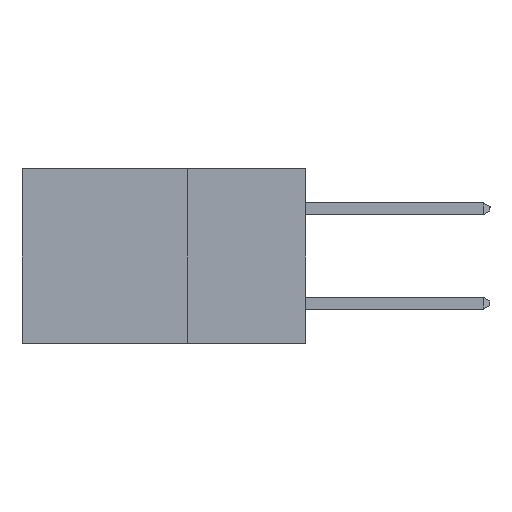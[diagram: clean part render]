
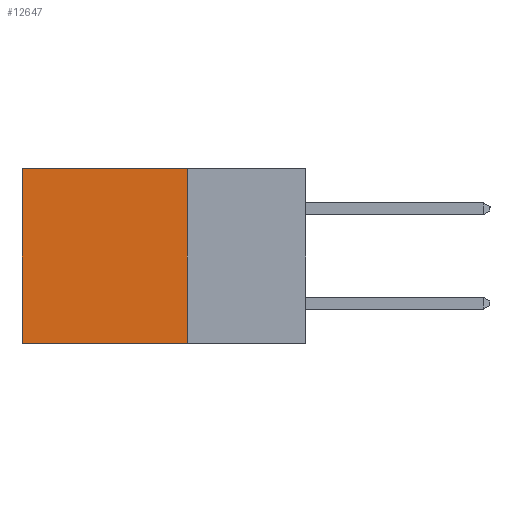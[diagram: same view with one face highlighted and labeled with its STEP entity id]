
A CAD part, left-side view. The second image highlights one B-rep face of the part: STEP entity #12647.
In plain terms, the highlighted planar face has unit normal (-1, 0, 0).
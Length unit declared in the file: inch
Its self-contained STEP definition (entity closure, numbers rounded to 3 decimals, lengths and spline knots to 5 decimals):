
#113 = CARTESIAN_POINT ( 'NONE',  ( 0.2615, 0.25, -0.37 ) ) ;
#217 = ORIENTED_EDGE ( 'NONE', *, *, #1676, .F. ) ;
#892 = LINE ( 'NONE', #4940, #4235 ) ;
#1184 = VERTEX_POINT ( 'NONE', #7299 ) ;
#1630 = DIRECTION ( 'NONE',  ( 0., 0., -1. ) ) ;
#1676 = EDGE_CURVE ( 'NONE', #11204, #1184, #4593, .T. ) ;
#1895 = EDGE_CURVE ( 'NONE', #12388, #11085, #5911, .T. ) ;
#1985 = LINE ( 'NONE', #113, #3358 ) ;
#2495 = DIRECTION ( 'NONE',  ( 1., 0., 0. ) ) ;
#2974 = ORIENTED_EDGE ( 'NONE', *, *, #5444, .F. ) ;
#3358 = VECTOR ( 'NONE', #10035, 39.37008 ) ;
#3526 = CARTESIAN_POINT ( 'NONE',  ( 0.2615, 0.25, -0.37 ) ) ;
#3724 = VECTOR ( 'NONE', #10959, 39.37008 ) ;
#3779 = CARTESIAN_POINT ( 'NONE',  ( 0.2615, 0.25, -0.37 ) ) ;
#4235 = VECTOR ( 'NONE', #12076, 39.37008 ) ;
#4593 = LINE ( 'NONE', #3526, #8417 ) ;
#4940 = CARTESIAN_POINT ( 'NONE',  ( 0.2615, 0.6, -0.37 ) ) ;
#5444 = EDGE_CURVE ( 'NONE', #12388, #11204, #1985, .T. ) ;
#5645 = EDGE_LOOP ( 'NONE', ( #9044, #217, #2974, #6342 ) ) ;
#5911 = LINE ( 'NONE', #6913, #3724 ) ;
#5971 = CARTESIAN_POINT ( 'NONE',  ( 0.2615, 0.25, 0. ) ) ;
#6342 = ORIENTED_EDGE ( 'NONE', *, *, #1895, .T. ) ;
#6505 = CARTESIAN_POINT ( 'NONE',  ( 0.2615, 0.25, -0.37 ) ) ;
#6913 = CARTESIAN_POINT ( 'NONE',  ( 0.2615, 0.25, 0. ) ) ;
#7299 = CARTESIAN_POINT ( 'NONE',  ( 0.2615, 0.6, -0.37 ) ) ;
#7710 = EDGE_CURVE ( 'NONE', #11085, #1184, #892, .T. ) ;
#8417 = VECTOR ( 'NONE', #9404, 39.37008 ) ;
#8607 = CARTESIAN_POINT ( 'NONE',  ( 0.2615, 0.6, 0. ) ) ;
#9044 = ORIENTED_EDGE ( 'NONE', *, *, #7710, .T. ) ;
#9404 = DIRECTION ( 'NONE',  ( 0., 1., 0. ) ) ;
#10035 = DIRECTION ( 'NONE',  ( 0., 0., -1. ) ) ;
#10548 = FACE_OUTER_BOUND ( 'NONE', #5645, .T. ) ;
#10959 = DIRECTION ( 'NONE',  ( 0., 1., 0. ) ) ;
#11085 = VERTEX_POINT ( 'NONE', #8607 ) ;
#11204 = VERTEX_POINT ( 'NONE', #3779 ) ;
#11752 = AXIS2_PLACEMENT_3D ( 'NONE', #6505, #2495, #1630 ) ;
#11764 = PLANE ( 'NONE',  #11752 ) ;
#12076 = DIRECTION ( 'NONE',  ( 0., 0., -1. ) ) ;
#12388 = VERTEX_POINT ( 'NONE', #5971 ) ;
#12647 = ADVANCED_FACE ( 'NONE', ( #10548 ), #11764, .F. ) ;
